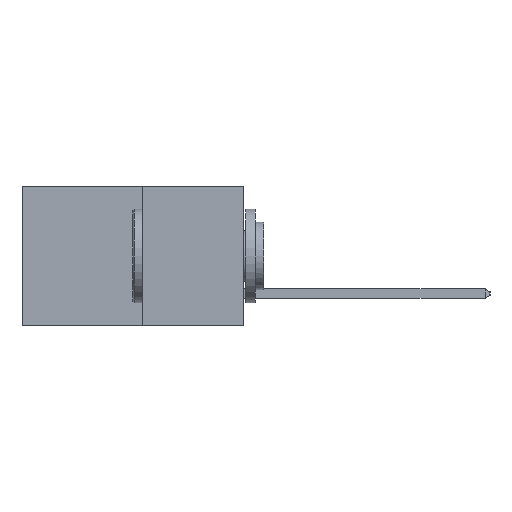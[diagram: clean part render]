
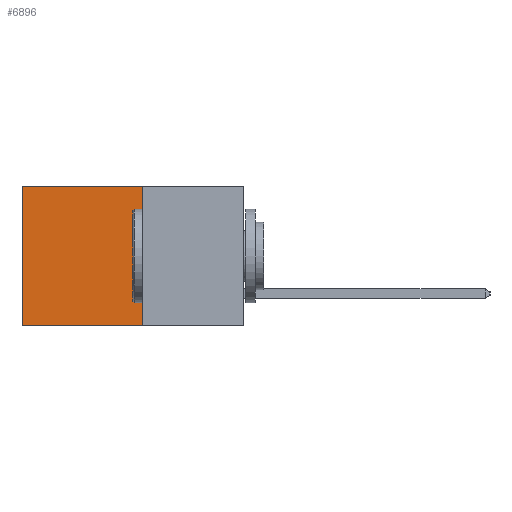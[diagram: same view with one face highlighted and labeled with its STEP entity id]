
A CAD part, left-side view. The second image highlights one B-rep face of the part: STEP entity #6896.
In plain terms, the highlighted planar face has unit normal (-1, 0, 0).
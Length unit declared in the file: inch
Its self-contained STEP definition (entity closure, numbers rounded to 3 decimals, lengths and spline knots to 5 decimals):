
#2006 = LINE ( 'NONE', #2983, #8142 ) ;
#2271 = CARTESIAN_POINT ( 'NONE',  ( 0.277, 0.27, -0.37 ) ) ;
#2289 = VERTEX_POINT ( 'NONE', #10041 ) ;
#2917 = VERTEX_POINT ( 'NONE', #7408 ) ;
#2983 = CARTESIAN_POINT ( 'NONE',  ( 0.277, 0.27, -0.37 ) ) ;
#3083 = LINE ( 'NONE', #7896, #9123 ) ;
#3319 = ORIENTED_EDGE ( 'NONE', *, *, #7435, .T. ) ;
#3345 = ORIENTED_EDGE ( 'NONE', *, *, #6492, .F. ) ;
#3359 = VERTEX_POINT ( 'NONE', #3371 ) ;
#3368 = ORIENTED_EDGE ( 'NONE', *, *, #9233, .F. ) ;
#3371 = CARTESIAN_POINT ( 'NONE',  ( 0.277, 0.59, -0.37 ) ) ;
#3806 = DIRECTION ( 'NONE',  ( 0., 1., 0. ) ) ;
#3823 = VECTOR ( 'NONE', #9340, 39.37008 ) ;
#3878 = VERTEX_POINT ( 'NONE', #10298 ) ;
#4729 = PLANE ( 'NONE',  #5498 ) ;
#4747 = LINE ( 'NONE', #5627, #8644 ) ;
#5015 = FACE_OUTER_BOUND ( 'NONE', #9684, .T. ) ;
#5323 = EDGE_CURVE ( 'NONE', #2289, #2917, #3083, .T. ) ;
#5498 = AXIS2_PLACEMENT_3D ( 'NONE', #2271, #10094, #5585 ) ;
#5522 = DIRECTION ( 'NONE',  ( 0., 0., -1. ) ) ;
#5585 = DIRECTION ( 'NONE',  ( 0., 0., -1. ) ) ;
#5627 = CARTESIAN_POINT ( 'NONE',  ( 0.277, 0.27, -0.37 ) ) ;
#6492 = EDGE_CURVE ( 'NONE', #2289, #3878, #4747, .T. ) ;
#6896 = ADVANCED_FACE ( 'NONE', ( #5015 ), #4729, .F. ) ;
#7103 = CARTESIAN_POINT ( 'NONE',  ( 0.277, 0.59, -0.37 ) ) ;
#7408 = CARTESIAN_POINT ( 'NONE',  ( 0.277, 0.59, 0. ) ) ;
#7435 = EDGE_CURVE ( 'NONE', #2917, #3359, #8312, .T. ) ;
#7674 = DIRECTION ( 'NONE',  ( 0., 1., 0. ) ) ;
#7896 = CARTESIAN_POINT ( 'NONE',  ( 0.277, 0.27, 0. ) ) ;
#8142 = VECTOR ( 'NONE', #3806, 39.37008 ) ;
#8312 = LINE ( 'NONE', #7103, #3823 ) ;
#8334 = ORIENTED_EDGE ( 'NONE', *, *, #5323, .T. ) ;
#8644 = VECTOR ( 'NONE', #5522, 39.37008 ) ;
#9123 = VECTOR ( 'NONE', #7674, 39.37008 ) ;
#9233 = EDGE_CURVE ( 'NONE', #3878, #3359, #2006, .T. ) ;
#9340 = DIRECTION ( 'NONE',  ( 0., 0., -1. ) ) ;
#9684 = EDGE_LOOP ( 'NONE', ( #3319, #3368, #3345, #8334 ) ) ;
#10041 = CARTESIAN_POINT ( 'NONE',  ( 0.277, 0.27, 0. ) ) ;
#10094 = DIRECTION ( 'NONE',  ( 1., 0., 0. ) ) ;
#10298 = CARTESIAN_POINT ( 'NONE',  ( 0.277, 0.27, -0.37 ) ) ;
